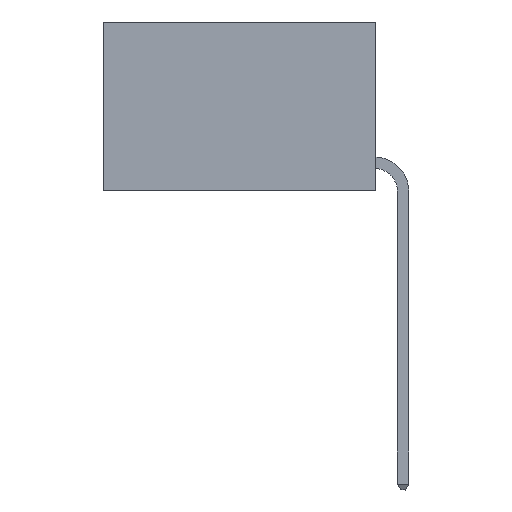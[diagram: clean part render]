
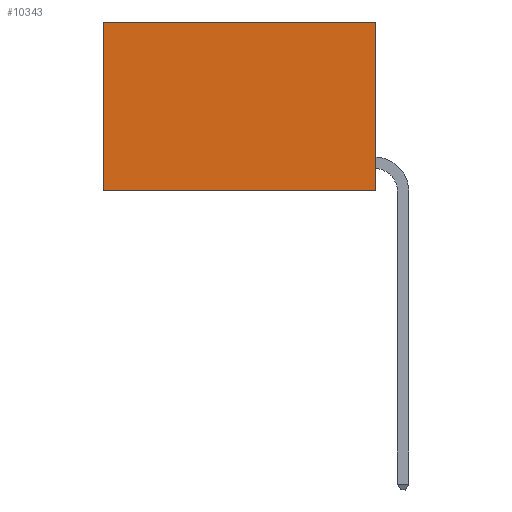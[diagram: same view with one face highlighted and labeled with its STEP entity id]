
A CAD part, left-side view. The second image highlights one B-rep face of the part: STEP entity #10343.
In plain terms, the highlighted planar face has unit normal (-1, 0, 0).
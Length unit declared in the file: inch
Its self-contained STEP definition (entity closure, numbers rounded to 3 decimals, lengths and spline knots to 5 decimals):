
#451 = EDGE_LOOP ( 'NONE', ( #11127, #11877, #1315, #4671 ) ) ;
#1119 = EDGE_CURVE ( 'NONE', #10717, #8027, #2012, .T. ) ;
#1315 = ORIENTED_EDGE ( 'NONE', *, *, #6425, .F. ) ;
#1650 = VECTOR ( 'NONE', #2049, 39.37008 ) ;
#1954 = LINE ( 'NONE', #8763, #1650 ) ;
#2012 = LINE ( 'NONE', #11492, #6741 ) ;
#2049 = DIRECTION ( 'NONE',  ( 0., 1., 0. ) ) ;
#2377 = DIRECTION ( 'NONE',  ( 0., 0., -1. ) ) ;
#3032 = LINE ( 'NONE', #10844, #10300 ) ;
#3234 = CARTESIAN_POINT ( 'NONE',  ( 0.2625, 0., 0. ) ) ;
#3319 = LINE ( 'NONE', #9679, #10576 ) ;
#3497 = EDGE_CURVE ( 'NONE', #11043, #10717, #1954, .T. ) ;
#4099 = CARTESIAN_POINT ( 'NONE',  ( 0.2625, 0., 0. ) ) ;
#4671 = ORIENTED_EDGE ( 'NONE', *, *, #3497, .T. ) ;
#4714 = CARTESIAN_POINT ( 'NONE',  ( 0.2625, 0.6, 0. ) ) ;
#5059 = DIRECTION ( 'NONE',  ( 0., 0., -1. ) ) ;
#5917 = CARTESIAN_POINT ( 'NONE',  ( 0.2625, 0.6, -0.37 ) ) ;
#5960 = PLANE ( 'NONE',  #10997 ) ;
#6291 = VERTEX_POINT ( 'NONE', #8820 ) ;
#6425 = EDGE_CURVE ( 'NONE', #11043, #6291, #3032, .T. ) ;
#6587 = DIRECTION ( 'NONE',  ( 0., 0., -1. ) ) ;
#6741 = VECTOR ( 'NONE', #6587, 39.37008 ) ;
#6833 = EDGE_CURVE ( 'NONE', #6291, #8027, #3319, .T. ) ;
#7548 = FACE_OUTER_BOUND ( 'NONE', #451, .T. ) ;
#8027 = VERTEX_POINT ( 'NONE', #5917 ) ;
#8763 = CARTESIAN_POINT ( 'NONE',  ( 0.2625, 0., 0. ) ) ;
#8820 = CARTESIAN_POINT ( 'NONE',  ( 0.2625, 0., -0.37 ) ) ;
#9679 = CARTESIAN_POINT ( 'NONE',  ( 0.2625, 0., -0.37 ) ) ;
#10300 = VECTOR ( 'NONE', #2377, 39.37008 ) ;
#10343 = ADVANCED_FACE ( 'NONE', ( #7548 ), #5960, .F. ) ;
#10576 = VECTOR ( 'NONE', #10604, 39.37008 ) ;
#10604 = DIRECTION ( 'NONE',  ( 0., 1., 0. ) ) ;
#10696 = DIRECTION ( 'NONE',  ( 1., 0., 0. ) ) ;
#10717 = VERTEX_POINT ( 'NONE', #4714 ) ;
#10844 = CARTESIAN_POINT ( 'NONE',  ( 0.2625, 0., 0. ) ) ;
#10997 = AXIS2_PLACEMENT_3D ( 'NONE', #4099, #10696, #5059 ) ;
#11043 = VERTEX_POINT ( 'NONE', #3234 ) ;
#11127 = ORIENTED_EDGE ( 'NONE', *, *, #1119, .T. ) ;
#11492 = CARTESIAN_POINT ( 'NONE',  ( 0.2625, 0.6, 0. ) ) ;
#11877 = ORIENTED_EDGE ( 'NONE', *, *, #6833, .F. ) ;
